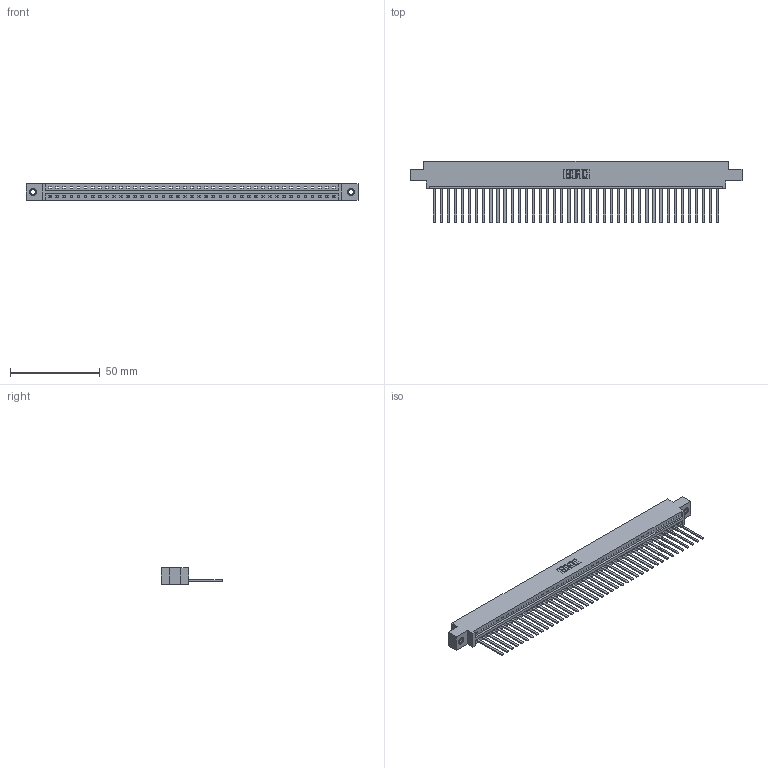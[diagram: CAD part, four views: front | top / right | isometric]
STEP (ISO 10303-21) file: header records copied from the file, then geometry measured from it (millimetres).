
FILE_DESCRIPTION (( 'STEP AP203' ), '1' );
FILE_NAME ('337-041-544-607.STEP', '2019-10-01T21:17:14', ( '' ), ( '' ), 'SwSTEP 2.0', 'SolidWorks 2016', '' );
FILE_SCHEMA (( 'CONFIG_CONTROL_DESIGN' ));
Length unit declared in the file: inch
Products named in the file (4): 345-292-001_345-293-144; 345-250-001_345-250-005-103; 337 Part_0.170 Offset - 0.156 Dia-TI; 337-041-544-607
Assembly tree (44 placements, depth 2):
  337-041-544-607
    337 Part_0.170 Offset - 0.156 Dia-TI
    345-292-001_345-293-144  x41
    345-250-001_345-250-005-103  x2
Bounding box: 185.47 x 34.3 x 9.4 mm (x, y, z)
Volume: 19607.9 mm3; surface area: 21955.8 mm2
Topology: 44 solids, 44 shells, 2474 faces, 7429 edges, 4890 vertices
Faces by surface type: plane 1828, cylinder 630, cone 12, torus 4
Entity records: 31740 total; most frequent: CARTESIAN_POINT 5508, ORIENTED_EDGE 5478, DIRECTION 4667, EDGE_CURVE 2739, LINE 2595, VECTOR 2595, VERTEX_POINT 1820, AXIS2_PLACEMENT_3D 1036
